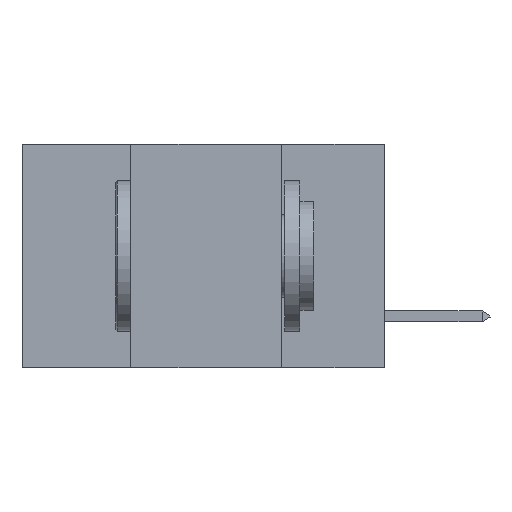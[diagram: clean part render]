
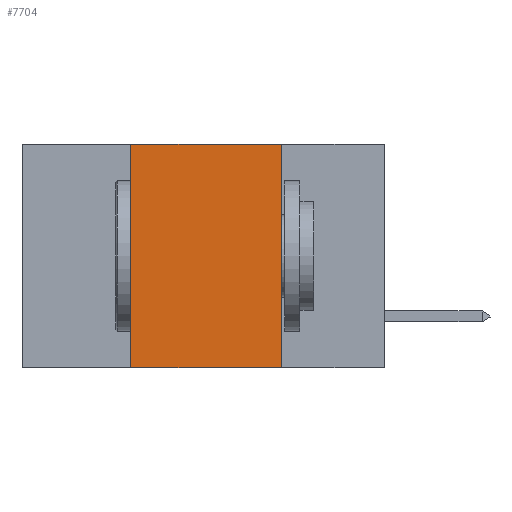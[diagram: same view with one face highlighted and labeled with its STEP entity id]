
A CAD part, left-side view. The second image highlights one B-rep face of the part: STEP entity #7704.
In plain terms, the highlighted planar face has unit normal (-1, 0, 0).
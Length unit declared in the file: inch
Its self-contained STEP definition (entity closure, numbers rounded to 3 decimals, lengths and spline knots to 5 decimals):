
#917 = VERTEX_POINT ( 'NONE', #3349 ) ;
#1912 = CARTESIAN_POINT ( 'NONE',  ( 0., 0.17, 0. ) ) ;
#1926 = DIRECTION ( 'NONE',  ( 0., -1., 0. ) ) ;
#2162 = DIRECTION ( 'NONE',  ( 0., 0., -1. ) ) ;
#2282 = LINE ( 'NONE', #2669, #6025 ) ;
#2669 = CARTESIAN_POINT ( 'NONE',  ( 0., 0.6, 0. ) ) ;
#2939 = DIRECTION ( 'NONE',  ( 0., -1., 0. ) ) ;
#2961 = EDGE_CURVE ( 'NONE', #7657, #917, #7182, .T. ) ;
#2985 = EDGE_CURVE ( 'NONE', #7657, #8722, #5682, .T. ) ;
#3106 = LINE ( 'NONE', #6597, #5211 ) ;
#3349 = CARTESIAN_POINT ( 'NONE',  ( 0., 0.42, 0. ) ) ;
#3810 = EDGE_CURVE ( 'NONE', #917, #7677, #2282, .T. ) ;
#3851 = AXIS2_PLACEMENT_3D ( 'NONE', #7137, #4226, #7879 ) ;
#4155 = EDGE_CURVE ( 'NONE', #7677, #8722, #3106, .T. ) ;
#4226 = DIRECTION ( 'NONE',  ( 1., 0., 0. ) ) ;
#4265 = ORIENTED_EDGE ( 'NONE', *, *, #3810, .F. ) ;
#4529 = ORIENTED_EDGE ( 'NONE', *, *, #2985, .T. ) ;
#4759 = VECTOR ( 'NONE', #7370, 39.37008 ) ;
#4993 = ORIENTED_EDGE ( 'NONE', *, *, #4155, .F. ) ;
#5156 = CARTESIAN_POINT ( 'NONE',  ( 0., 0.42, 0. ) ) ;
#5211 = VECTOR ( 'NONE', #2162, 39.37008 ) ;
#5540 = ORIENTED_EDGE ( 'NONE', *, *, #2961, .F. ) ;
#5682 = LINE ( 'NONE', #8830, #7633 ) ;
#6025 = VECTOR ( 'NONE', #1926, 39.37008 ) ;
#6028 = EDGE_LOOP ( 'NONE', ( #4993, #4265, #5540, #4529 ) ) ;
#6328 = FACE_OUTER_BOUND ( 'NONE', #6028, .T. ) ;
#6597 = CARTESIAN_POINT ( 'NONE',  ( 0., 0.17, 0. ) ) ;
#7137 = CARTESIAN_POINT ( 'NONE',  ( 0., 0.6, 0. ) ) ;
#7182 = LINE ( 'NONE', #5156, #4759 ) ;
#7370 = DIRECTION ( 'NONE',  ( 0., 0., 1. ) ) ;
#7444 = CARTESIAN_POINT ( 'NONE',  ( 0., 0.17, -0.37 ) ) ;
#7633 = VECTOR ( 'NONE', #2939, 39.37008 ) ;
#7657 = VERTEX_POINT ( 'NONE', #8556 ) ;
#7677 = VERTEX_POINT ( 'NONE', #1912 ) ;
#7704 = ADVANCED_FACE ( 'NONE', ( #6328 ), #7844, .F. ) ;
#7844 = PLANE ( 'NONE',  #3851 ) ;
#7879 = DIRECTION ( 'NONE',  ( 0., 0., -1. ) ) ;
#8556 = CARTESIAN_POINT ( 'NONE',  ( 0., 0.42, -0.37 ) ) ;
#8722 = VERTEX_POINT ( 'NONE', #7444 ) ;
#8830 = CARTESIAN_POINT ( 'NONE',  ( 0., 0.6, -0.37 ) ) ;
